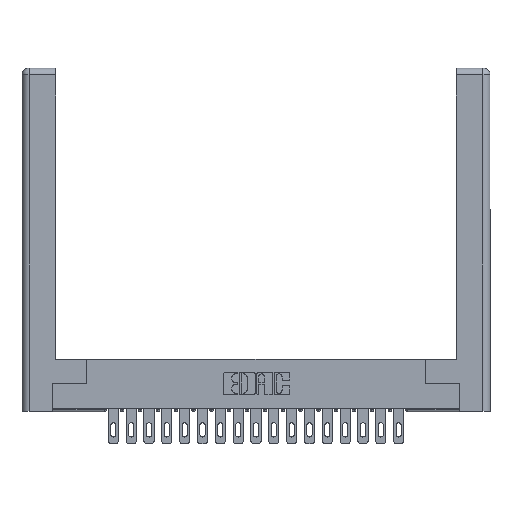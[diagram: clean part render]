
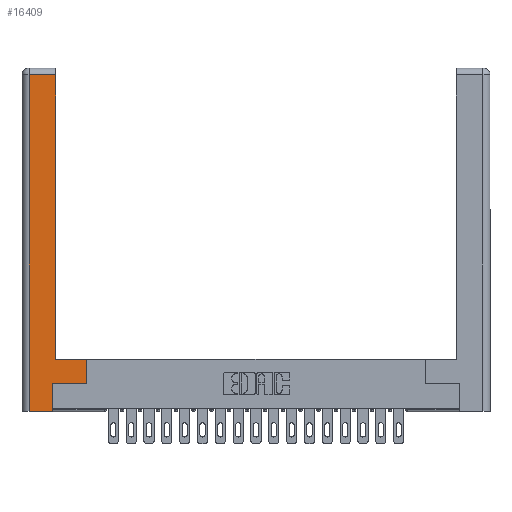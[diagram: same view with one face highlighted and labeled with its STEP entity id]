
A CAD part, top view. The second image highlights one B-rep face of the part: STEP entity #16409.
In plain terms, the highlighted planar face has unit normal (0, 0, 1).
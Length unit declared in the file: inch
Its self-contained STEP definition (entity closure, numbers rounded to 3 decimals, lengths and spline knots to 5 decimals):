
#119 = CARTESIAN_POINT ( 'NONE',  ( 0.565, 0.45, 0. ) ) ;
#191 = VERTEX_POINT ( 'NONE', #18947 ) ;
#911 = VERTEX_POINT ( 'NONE', #7703 ) ;
#1302 = CARTESIAN_POINT ( 'NONE',  ( 0.265, 0.245, 0. ) ) ;
#2163 = VECTOR ( 'NONE', #9771, 39.37008 ) ;
#2556 = VECTOR ( 'NONE', #18388, 39.37008 ) ;
#2833 = DIRECTION ( 'NONE',  ( 0., -1., 0. ) ) ;
#3243 = VERTEX_POINT ( 'NONE', #119 ) ;
#3809 = EDGE_CURVE ( 'NONE', #18143, #14297, #22626, .T. ) ;
#4110 = VERTEX_POINT ( 'NONE', #5234 ) ;
#4132 = ORIENTED_EDGE ( 'NONE', *, *, #15574, .T. ) ;
#5092 = EDGE_CURVE ( 'NONE', #3243, #18143, #14985, .T. ) ;
#5195 = CARTESIAN_POINT ( 'NONE',  ( 0.565, 0.45, 0. ) ) ;
#5219 = FACE_OUTER_BOUND ( 'NONE', #20503, .T. ) ;
#5234 = CARTESIAN_POINT ( 'NONE',  ( 0.265, 0., 0. ) ) ;
#5572 = VECTOR ( 'NONE', #11312, 39.37008 ) ;
#6514 = LINE ( 'NONE', #22324, #10916 ) ;
#6641 = VECTOR ( 'NONE', #2833, 39.37008 ) ;
#6731 = PLANE ( 'NONE',  #18588 ) ;
#7015 = CARTESIAN_POINT ( 'NONE',  ( 0.0615, 0., 0. ) ) ;
#7357 = CARTESIAN_POINT ( 'NONE',  ( 0.565, 0.245, 0. ) ) ;
#7361 = ORIENTED_EDGE ( 'NONE', *, *, #15233, .T. ) ;
#7703 = CARTESIAN_POINT ( 'NONE',  ( 0.0615, 2.94, 0. ) ) ;
#7728 = CARTESIAN_POINT ( 'NONE',  ( 0.295, 0.45, 0. ) ) ;
#8202 = ORIENTED_EDGE ( 'NONE', *, *, #3809, .T. ) ;
#8263 = ORIENTED_EDGE ( 'NONE', *, *, #5092, .T. ) ;
#8541 = ORIENTED_EDGE ( 'NONE', *, *, #8616, .T. ) ;
#8616 = EDGE_CURVE ( 'NONE', #191, #3243, #10452, .T. ) ;
#8625 = DIRECTION ( 'NONE',  ( 0., 0., -1. ) ) ;
#9136 = ORIENTED_EDGE ( 'NONE', *, *, #20626, .T. ) ;
#9693 = CARTESIAN_POINT ( 'NONE',  ( 0.265, 0.245, 0. ) ) ;
#9771 = DIRECTION ( 'NONE',  ( -1., 0., 0. ) ) ;
#10452 = LINE ( 'NONE', #5195, #2556 ) ;
#10513 = DIRECTION ( 'NONE',  ( -1., 0., 0. ) ) ;
#10911 = DIRECTION ( 'NONE',  ( 0., 1., 0. ) ) ;
#10916 = VECTOR ( 'NONE', #18459, 39.37008 ) ;
#11312 = DIRECTION ( 'NONE',  ( 0., 1., 0. ) ) ;
#12726 = EDGE_CURVE ( 'NONE', #23288, #191, #13237, .T. ) ;
#13237 = LINE ( 'NONE', #7357, #20788 ) ;
#13339 = EDGE_CURVE ( 'NONE', #13387, #4110, #13762, .T. ) ;
#13387 = VERTEX_POINT ( 'NONE', #7015 ) ;
#13550 = ORIENTED_EDGE ( 'NONE', *, *, #12726, .T. ) ;
#13762 = LINE ( 'NONE', #22098, #20179 ) ;
#14056 = CARTESIAN_POINT ( 'NONE',  ( 0.0615, 0., 0. ) ) ;
#14297 = VERTEX_POINT ( 'NONE', #19123 ) ;
#14618 = DIRECTION ( 'NONE',  ( 1., 0., 0. ) ) ;
#14645 = ORIENTED_EDGE ( 'NONE', *, *, #13339, .T. ) ;
#14658 = CARTESIAN_POINT ( 'NONE',  ( 0.295, 3., 0. ) ) ;
#14911 = LINE ( 'NONE', #9693, #5572 ) ;
#14985 = LINE ( 'NONE', #7728, #2163 ) ;
#15233 = EDGE_CURVE ( 'NONE', #911, #13387, #20952, .T. ) ;
#15574 = EDGE_CURVE ( 'NONE', #4110, #23288, #14911, .T. ) ;
#16191 = VECTOR ( 'NONE', #10911, 39.37008 ) ;
#16409 = ADVANCED_FACE ( 'NONE', ( #5219 ), #6731, .F. ) ;
#17388 = CARTESIAN_POINT ( 'NONE',  ( 0.295, 0.45, 0. ) ) ;
#18143 = VERTEX_POINT ( 'NONE', #17388 ) ;
#18388 = DIRECTION ( 'NONE',  ( 0., 1., 0. ) ) ;
#18459 = DIRECTION ( 'NONE',  ( -1., 0., 0. ) ) ;
#18588 = AXIS2_PLACEMENT_3D ( 'NONE', #19730, #8625, #10513 ) ;
#18947 = CARTESIAN_POINT ( 'NONE',  ( 0.565, 0.245, 0. ) ) ;
#19123 = CARTESIAN_POINT ( 'NONE',  ( 0.295, 2.94, 0. ) ) ;
#19730 = CARTESIAN_POINT ( 'NONE',  ( 0., 0., 0. ) ) ;
#20179 = VECTOR ( 'NONE', #14618, 39.37008 ) ;
#20503 = EDGE_LOOP ( 'NONE', ( #8202, #9136, #7361, #14645, #4132, #13550, #8541, #8263 ) ) ;
#20562 = DIRECTION ( 'NONE',  ( 1., 0., 0. ) ) ;
#20626 = EDGE_CURVE ( 'NONE', #14297, #911, #6514, .T. ) ;
#20788 = VECTOR ( 'NONE', #20562, 39.37008 ) ;
#20952 = LINE ( 'NONE', #14056, #6641 ) ;
#22098 = CARTESIAN_POINT ( 'NONE',  ( 0.265, 0., 0. ) ) ;
#22324 = CARTESIAN_POINT ( 'NONE',  ( 0.0615, 2.94, 0. ) ) ;
#22626 = LINE ( 'NONE', #14658, #16191 ) ;
#23288 = VERTEX_POINT ( 'NONE', #1302 ) ;
